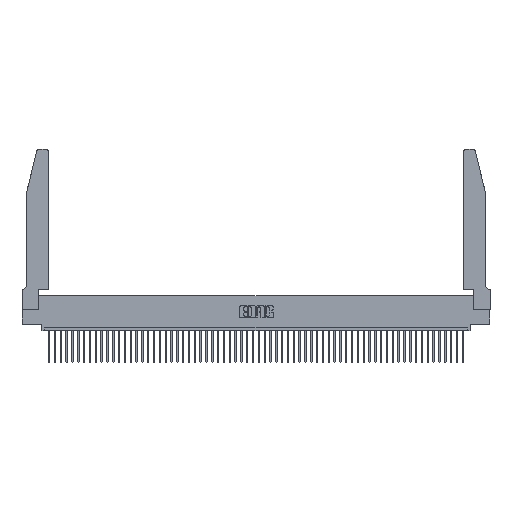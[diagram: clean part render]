
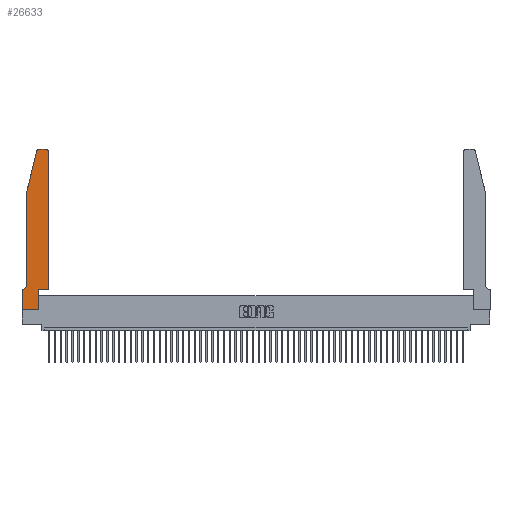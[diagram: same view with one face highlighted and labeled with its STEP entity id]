
A CAD part, top view. The second image highlights one B-rep face of the part: STEP entity #26633.
In plain terms, the highlighted planar face has unit normal (0, 0, 1).
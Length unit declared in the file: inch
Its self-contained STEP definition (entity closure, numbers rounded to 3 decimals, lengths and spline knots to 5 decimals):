
#639 = ORIENTED_EDGE ( 'NONE', *, *, #11816, .T. ) ;
#1179 = DIRECTION ( 'NONE',  ( 0., 0., 1. ) ) ;
#1491 = ORIENTED_EDGE ( 'NONE', *, *, #53139, .T. ) ;
#1664 = DIRECTION ( 'NONE',  ( -1., 0., 0. ) ) ;
#1717 = LINE ( 'NONE', #40835, #10343 ) ;
#2142 = DIRECTION ( 'NONE',  ( 1., 0., 0. ) ) ;
#2210 = DIRECTION ( 'NONE',  ( 1., 0., 0. ) ) ;
#3397 = ORIENTED_EDGE ( 'NONE', *, *, #37651, .T. ) ;
#3454 = CARTESIAN_POINT ( 'NONE',  ( 0.284, 2.75, 0.37 ) ) ;
#4113 = EDGE_CURVE ( 'NONE', #29719, #28272, #33433, .T. ) ;
#4260 = ORIENTED_EDGE ( 'NONE', *, *, #23999, .T. ) ;
#4776 = VECTOR ( 'NONE', #35150, 39.37008 ) ;
#6139 = CARTESIAN_POINT ( 'NONE',  ( 0.4505, 0.35, 0.37 ) ) ;
#6194 = CARTESIAN_POINT ( 'NONE',  ( 0.0755, 0.35, 0.37 ) ) ;
#6736 = LINE ( 'NONE', #11413, #13298 ) ;
#6829 = EDGE_CURVE ( 'NONE', #52606, #33632, #14346, .T. ) ;
#7781 = CIRCLE ( 'NONE', #19334, 0.03 ) ;
#8702 = VERTEX_POINT ( 'NONE', #45390 ) ;
#9130 = CARTESIAN_POINT ( 'NONE',  ( 0.4505, 0.35, 0.37 ) ) ;
#9767 = EDGE_CURVE ( 'NONE', #34080, #13189, #45319, .T. ) ;
#10343 = VECTOR ( 'NONE', #22119, 39.37008 ) ;
#10820 = DIRECTION ( 'NONE',  ( -1., 0., 0. ) ) ;
#11413 = CARTESIAN_POINT ( 'NONE',  ( 0.0755, 2., 0.37 ) ) ;
#11816 = EDGE_CURVE ( 'NONE', #28272, #47354, #7781, .T. ) ;
#12551 = LINE ( 'NONE', #35647, #35115 ) ;
#13189 = VERTEX_POINT ( 'NONE', #39993 ) ;
#13247 = CIRCLE ( 'NONE', #30739, 0.03 ) ;
#13298 = VECTOR ( 'NONE', #53614, 39.37008 ) ;
#14346 = CIRCLE ( 'NONE', #20246, 0.07 ) ;
#14390 = LINE ( 'NONE', #26247, #39670 ) ;
#15393 = CARTESIAN_POINT ( 'NONE',  ( 0.4205, 2.75, 0.37 ) ) ;
#18864 = ORIENTED_EDGE ( 'NONE', *, *, #45995, .T. ) ;
#19334 = AXIS2_PLACEMENT_3D ( 'NONE', #44142, #39954, #25310 ) ;
#19336 = VECTOR ( 'NONE', #24495, 39.37008 ) ;
#19430 = CARTESIAN_POINT ( 'NONE',  ( 0.0755, 2., 0.37 ) ) ;
#19854 = DIRECTION ( 'NONE',  ( 0., -1., 0. ) ) ;
#20246 = AXIS2_PLACEMENT_3D ( 'NONE', #24998, #21390, #25712 ) ;
#20575 = ORIENTED_EDGE ( 'NONE', *, *, #9767, .T. ) ;
#20758 = ORIENTED_EDGE ( 'NONE', *, *, #27067, .T. ) ;
#21089 = FACE_OUTER_BOUND ( 'NONE', #52417, .T. ) ;
#21356 = EDGE_CURVE ( 'NONE', #47354, #25982, #14390, .T. ) ;
#21390 = DIRECTION ( 'NONE',  ( 0., 0., -1. ) ) ;
#21460 = CARTESIAN_POINT ( 'NONE',  ( 0.2865, 0., 0.37 ) ) ;
#21694 = VECTOR ( 'NONE', #32976, 39.37008 ) ;
#22119 = DIRECTION ( 'NONE',  ( -0.239, -0.971, 0. ) ) ;
#22178 = CARTESIAN_POINT ( 'NONE',  ( 0., 0.35, 0.37 ) ) ;
#22360 = PLANE ( 'NONE',  #37531 ) ;
#23266 = VECTOR ( 'NONE', #2210, 39.37008 ) ;
#23999 = EDGE_CURVE ( 'NONE', #32691, #52606, #6736, .T. ) ;
#24495 = DIRECTION ( 'NONE',  ( 0., 1., 0. ) ) ;
#24998 = CARTESIAN_POINT ( 'NONE',  ( 0.0055, 0.42, 0.37 ) ) ;
#25310 = DIRECTION ( 'NONE',  ( 1., 0., 0. ) ) ;
#25712 = DIRECTION ( 'NONE',  ( -1., 0., 0. ) ) ;
#25913 = ORIENTED_EDGE ( 'NONE', *, *, #21356, .T. ) ;
#25982 = VERTEX_POINT ( 'NONE', #3454 ) ;
#26247 = CARTESIAN_POINT ( 'NONE',  ( 0.2605, 2.75, 0.37 ) ) ;
#26633 = ADVANCED_FACE ( 'NONE', ( #21089 ), #22360, .T. ) ;
#26866 = CARTESIAN_POINT ( 'NONE',  ( 0., 0., 0.37 ) ) ;
#27067 = EDGE_CURVE ( 'NONE', #44236, #34080, #34385, .T. ) ;
#27353 = VERTEX_POINT ( 'NONE', #54951 ) ;
#28272 = VERTEX_POINT ( 'NONE', #33911 ) ;
#29719 = VERTEX_POINT ( 'NONE', #6139 ) ;
#30124 = CARTESIAN_POINT ( 'NONE',  ( 0.0055, 0.35, 0.37 ) ) ;
#30739 = AXIS2_PLACEMENT_3D ( 'NONE', #47529, #1179, #2142 ) ;
#32691 = VERTEX_POINT ( 'NONE', #19430 ) ;
#32976 = DIRECTION ( 'NONE',  ( 1., 0., 0. ) ) ;
#33433 = LINE ( 'NONE', #9130, #4776 ) ;
#33632 = VERTEX_POINT ( 'NONE', #30124 ) ;
#33911 = CARTESIAN_POINT ( 'NONE',  ( 0.4505, 2.72, 0.37 ) ) ;
#34080 = VERTEX_POINT ( 'NONE', #21460 ) ;
#34385 = LINE ( 'NONE', #36682, #21694 ) ;
#35055 = DIRECTION ( 'NONE',  ( 1., 0., 0. ) ) ;
#35115 = VECTOR ( 'NONE', #19854, 39.37008 ) ;
#35150 = DIRECTION ( 'NONE',  ( 0., 1., 0. ) ) ;
#35247 = ORIENTED_EDGE ( 'NONE', *, *, #6829, .T. ) ;
#35647 = CARTESIAN_POINT ( 'NONE',  ( 0., 0., 0.37 ) ) ;
#36682 = CARTESIAN_POINT ( 'NONE',  ( 0., 0., 0.37 ) ) ;
#37345 = LINE ( 'NONE', #44625, #23266 ) ;
#37531 = AXIS2_PLACEMENT_3D ( 'NONE', #22178, #48254, #35055 ) ;
#37651 = EDGE_CURVE ( 'NONE', #8702, #32691, #1717, .T. ) ;
#39670 = VECTOR ( 'NONE', #1664, 39.37008 ) ;
#39954 = DIRECTION ( 'NONE',  ( 0., 0., 1. ) ) ;
#39993 = CARTESIAN_POINT ( 'NONE',  ( 0.2865, 0.35, 0.37 ) ) ;
#40655 = EDGE_CURVE ( 'NONE', #33632, #27353, #50709, .T. ) ;
#40835 = CARTESIAN_POINT ( 'NONE',  ( 0.0755, 2., 0.37 ) ) ;
#41821 = EDGE_CURVE ( 'NONE', #25982, #8702, #13247, .T. ) ;
#44142 = CARTESIAN_POINT ( 'NONE',  ( 0.4205, 2.72, 0.37 ) ) ;
#44236 = VERTEX_POINT ( 'NONE', #26866 ) ;
#44625 = CARTESIAN_POINT ( 'NONE',  ( 0.4505, 0.35, 0.37 ) ) ;
#45319 = LINE ( 'NONE', #53669, #19336 ) ;
#45390 = CARTESIAN_POINT ( 'NONE',  ( 0.25487, 2.72718, 0.37 ) ) ;
#45833 = CARTESIAN_POINT ( 'NONE',  ( 0.0755, 0.42, 0.37 ) ) ;
#45995 = EDGE_CURVE ( 'NONE', #27353, #44236, #12551, .T. ) ;
#47354 = VERTEX_POINT ( 'NONE', #15393 ) ;
#47529 = CARTESIAN_POINT ( 'NONE',  ( 0.284, 2.72, 0.37 ) ) ;
#48254 = DIRECTION ( 'NONE',  ( 0., 0., 1. ) ) ;
#48801 = ORIENTED_EDGE ( 'NONE', *, *, #41821, .T. ) ;
#50709 = LINE ( 'NONE', #6194, #51957 ) ;
#51219 = ORIENTED_EDGE ( 'NONE', *, *, #40655, .T. ) ;
#51928 = ORIENTED_EDGE ( 'NONE', *, *, #4113, .T. ) ;
#51957 = VECTOR ( 'NONE', #10820, 39.37008 ) ;
#52417 = EDGE_LOOP ( 'NONE', ( #25913, #48801, #3397, #4260, #35247, #51219, #18864, #20758, #20575, #1491, #51928, #639 ) ) ;
#52606 = VERTEX_POINT ( 'NONE', #45833 ) ;
#53139 = EDGE_CURVE ( 'NONE', #13189, #29719, #37345, .T. ) ;
#53614 = DIRECTION ( 'NONE',  ( 0., -1., 0. ) ) ;
#53669 = CARTESIAN_POINT ( 'NONE',  ( 0.2865, 0.35, 0.37 ) ) ;
#54951 = CARTESIAN_POINT ( 'NONE',  ( 0., 0.35, 0.37 ) ) ;
